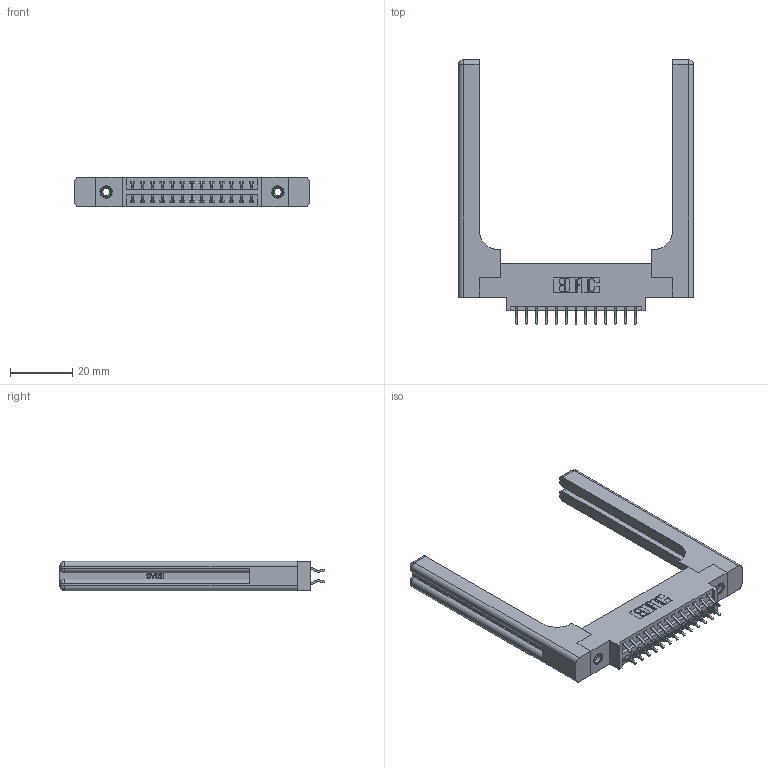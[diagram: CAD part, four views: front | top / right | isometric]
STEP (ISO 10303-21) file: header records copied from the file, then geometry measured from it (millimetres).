
FILE_DESCRIPTION (( 'STEP AP203' ), '1' );
FILE_NAME ('396-026-556-858.STEP', '2019-11-01T19:12:12', ( '' ), ( '' ), 'SwSTEP 2.0', 'SolidWorks 2016', '' );
FILE_SCHEMA (( 'CONFIG_CONTROL_DESIGN' ));
Length unit declared in the file: inch
Products named in the file (5): 346 Part_0.170 Offset - 0.156 Dia-TH; 345-292-001_556 Tail; 345-250-001_345-250-001-102; 346-220-058_345-220-058; 396-026-556-858
Assembly tree (31 placements, depth 2):
  396-026-556-858
    346 Part_0.170 Offset - 0.156 Dia-TH
    345-292-001_556 Tail  x26
    345-250-001_345-250-001-102  x2
    346-220-058_345-220-058  x2
Bounding box: 75.34 x 84.84 x 9.4 mm (x, y, z)
Volume: 14459.6 mm3; surface area: 14246.8 mm2
Topology: 31 solids, 31 shells, 1890 faces, 5505 edges, 3614 vertices
Faces by surface type: plane 1242, cylinder 588, bspline 36, cone 12, sphere 8, torus 4
Entity records: 17922 total; most frequent: CARTESIAN_POINT 4017, ORIENTED_EDGE 2736, DIRECTION 2512, EDGE_CURVE 1368, VECTOR 1084, LINE 1084, VERTEX_POINT 902, AXIS2_PLACEMENT_3D 714
